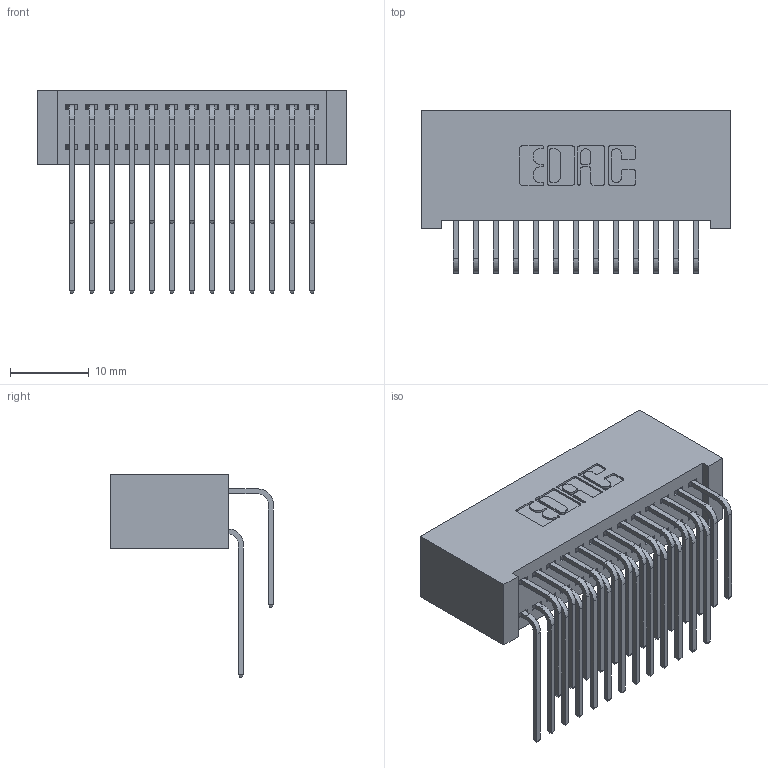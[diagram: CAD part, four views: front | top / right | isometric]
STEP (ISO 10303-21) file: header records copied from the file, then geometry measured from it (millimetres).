
FILE_DESCRIPTION (( 'STEP AP203' ), '1' );
FILE_NAME ('342-026-559-201.STEP', '2018-08-11T05:14:26', ( '' ), ( '' ), 'SwSTEP 2.0', 'SolidWorks 2016', '' );
FILE_SCHEMA (( 'CONFIG_CONTROL_DESIGN' ));
Length unit declared in the file: inch
Products named in the file (4): 342-026-559-201; 342 Part_Lugless; 345-292-001_558 559 Tail - 1; 345-292-001_559 Tail - 2
Assembly tree (27 placements, depth 2):
  342-026-559-201
    342 Part_Lugless
    345-292-001_558 559 Tail - 1  x13
    345-292-001_559 Tail - 2  x13
Bounding box: 39.27 x 20.64 x 25.78 mm (x, y, z)
Volume: 3980.5 mm3; surface area: 6889.4 mm2
Topology: 27 solids, 27 shells, 1506 faces, 4461 edges, 2938 vertices
Faces by surface type: plane 1050, cylinder 456
Entity records: 13489 total; most frequent: CARTESIAN_POINT 2317, ORIENTED_EDGE 2202, DIRECTION 2005, EDGE_CURVE 1101, LINE 941, VECTOR 941, VERTEX_POINT 730, AXIS2_PLACEMENT_3D 532
